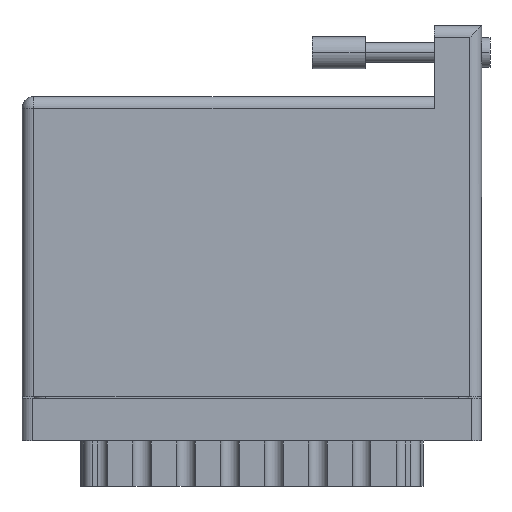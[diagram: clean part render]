
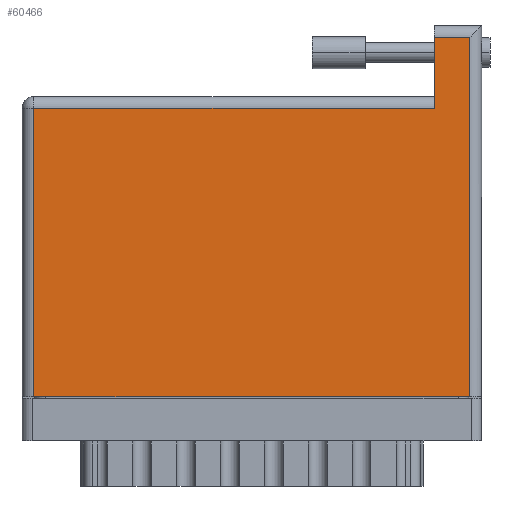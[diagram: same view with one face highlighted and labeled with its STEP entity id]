
A CAD part, front view. The second image highlights one B-rep face of the part: STEP entity #60466.
In plain terms, the highlighted face is planar.
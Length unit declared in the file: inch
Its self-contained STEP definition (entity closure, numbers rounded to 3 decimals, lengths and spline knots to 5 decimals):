
#2752 = ORIENTED_EDGE ( 'NONE', *, *, #30310, .T. ) ;
#3177 = ORIENTED_EDGE ( 'NONE', *, *, #24922, .T. ) ;
#4172 = VECTOR ( 'NONE', #41818, 39.37008 ) ;
#4535 = ORIENTED_EDGE ( 'NONE', *, *, #49325, .T. ) ;
#4813 = DIRECTION ( 'NONE',  ( 0., 0., -1. ) ) ;
#6298 = VECTOR ( 'NONE', #13498, 39.37008 ) ;
#11036 = CARTESIAN_POINT ( 'NONE',  ( 2.648, 2.125, 0. ) ) ;
#11369 = CARTESIAN_POINT ( 'NONE',  ( 0.07, 0., 0. ) ) ;
#12021 = VERTEX_POINT ( 'NONE', #60478 ) ;
#13050 = CARTESIAN_POINT ( 'NONE',  ( 0., 1.705, 0. ) ) ;
#13060 = FACE_OUTER_BOUND ( 'NONE', #62060, .T. ) ;
#13498 = DIRECTION ( 'NONE',  ( 0., 1., 0. ) ) ;
#15547 = CARTESIAN_POINT ( 'NONE',  ( 0., 1.775, 0. ) ) ;
#18668 = EDGE_CURVE ( 'NONE', #32365, #63389, #57829, .T. ) ;
#22556 = CARTESIAN_POINT ( 'NONE',  ( 0.07, 1.705, 0. ) ) ;
#24429 = VECTOR ( 'NONE', #60510, 39.37008 ) ;
#24715 = VERTEX_POINT ( 'NONE', #58634 ) ;
#24922 = EDGE_CURVE ( 'NONE', #42735, #32036, #28645, .T. ) ;
#26894 = EDGE_CURVE ( 'NONE', #12021, #32365, #46437, .T. ) ;
#28645 = LINE ( 'NONE', #11369, #24429 ) ;
#30310 = EDGE_CURVE ( 'NONE', #63389, #24715, #46027, .T. ) ;
#32036 = VERTEX_POINT ( 'NONE', #51907 ) ;
#32365 = VERTEX_POINT ( 'NONE', #11036 ) ;
#38327 = ORIENTED_EDGE ( 'NONE', *, *, #59907, .T. ) ;
#41299 = VECTOR ( 'NONE', #45488, 39.37008 ) ;
#41580 = VECTOR ( 'NONE', #70280, 39.37008 ) ;
#41818 = DIRECTION ( 'NONE',  ( 0., -1., 0. ) ) ;
#42052 = DIRECTION ( 'NONE',  ( 1., 0., 0. ) ) ;
#42735 = VERTEX_POINT ( 'NONE', #22556 ) ;
#43185 = PLANE ( 'NONE',  #45512 ) ;
#43529 = CARTESIAN_POINT ( 'NONE',  ( 0., 2.125, 0. ) ) ;
#45488 = DIRECTION ( 'NONE',  ( -1., 0., 0. ) ) ;
#45512 = AXIS2_PLACEMENT_3D ( 'NONE', #15547, #4813, #64246 ) ;
#46027 = LINE ( 'NONE', #69281, #4172 ) ;
#46437 = LINE ( 'NONE', #51929, #6298 ) ;
#49325 = EDGE_CURVE ( 'NONE', #32036, #12021, #65035, .T. ) ;
#50710 = LINE ( 'NONE', #13050, #41299 ) ;
#51907 = CARTESIAN_POINT ( 'NONE',  ( 0.07, 0., 0. ) ) ;
#51929 = CARTESIAN_POINT ( 'NONE',  ( 2.648, 2.195, 0. ) ) ;
#57829 = LINE ( 'NONE', #43529, #41580 ) ;
#58155 = ORIENTED_EDGE ( 'NONE', *, *, #26894, .T. ) ;
#58634 = CARTESIAN_POINT ( 'NONE',  ( 2.438, 1.705, 0. ) ) ;
#59007 = CARTESIAN_POINT ( 'NONE',  ( 0., 0., 0. ) ) ;
#59907 = EDGE_CURVE ( 'NONE', #24715, #42735, #50710, .T. ) ;
#60466 = ADVANCED_FACE ( 'NONE', ( #13060 ), #43185, .F. ) ;
#60478 = CARTESIAN_POINT ( 'NONE',  ( 2.648, 0., 0. ) ) ;
#60510 = DIRECTION ( 'NONE',  ( 0., -1., 0. ) ) ;
#60777 = VECTOR ( 'NONE', #42052, 39.37008 ) ;
#62060 = EDGE_LOOP ( 'NONE', ( #38327, #3177, #4535, #58155, #63978, #2752 ) ) ;
#62660 = CARTESIAN_POINT ( 'NONE',  ( 2.438, 2.125, 0. ) ) ;
#63389 = VERTEX_POINT ( 'NONE', #62660 ) ;
#63978 = ORIENTED_EDGE ( 'NONE', *, *, #18668, .T. ) ;
#64246 = DIRECTION ( 'NONE',  ( -1., 0., 0. ) ) ;
#65035 = LINE ( 'NONE', #59007, #60777 ) ;
#69281 = CARTESIAN_POINT ( 'NONE',  ( 2.438, 2.195, 0. ) ) ;
#70280 = DIRECTION ( 'NONE',  ( -1., 0., 0. ) ) ;
